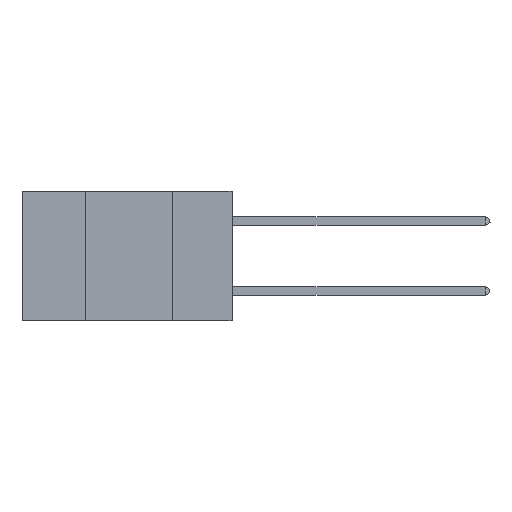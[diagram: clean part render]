
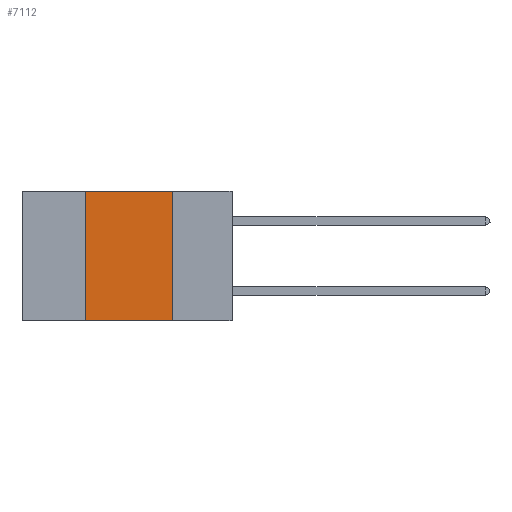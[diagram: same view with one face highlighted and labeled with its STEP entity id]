
A CAD part, left-side view. The second image highlights one B-rep face of the part: STEP entity #7112.
In plain terms, the highlighted planar face has unit normal (-1, 0, 0).
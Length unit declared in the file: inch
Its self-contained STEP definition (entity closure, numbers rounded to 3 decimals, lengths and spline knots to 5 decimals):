
#1137 = ORIENTED_EDGE ( 'NONE', *, *, #18672, .F. ) ;
#1663 = VERTEX_POINT ( 'NONE', #9083 ) ;
#2869 = VERTEX_POINT ( 'NONE', #22920 ) ;
#3941 = DIRECTION ( 'NONE',  ( 1., 0., 0. ) ) ;
#5808 = PLANE ( 'NONE',  #6796 ) ;
#6336 = CARTESIAN_POINT ( 'NONE',  ( 0., 0.42, 0. ) ) ;
#6553 = DIRECTION ( 'NONE',  ( 0., -1., 0. ) ) ;
#6796 = AXIS2_PLACEMENT_3D ( 'NONE', #20015, #3941, #12505 ) ;
#7112 = ADVANCED_FACE ( 'NONE', ( #7330 ), #5808, .F. ) ;
#7273 = LINE ( 'NONE', #19848, #7962 ) ;
#7315 = ORIENTED_EDGE ( 'NONE', *, *, #9141, .F. ) ;
#7330 = FACE_OUTER_BOUND ( 'NONE', #13004, .T. ) ;
#7962 = VECTOR ( 'NONE', #14661, 39.37008 ) ;
#8351 = VERTEX_POINT ( 'NONE', #16168 ) ;
#9083 = CARTESIAN_POINT ( 'NONE',  ( 0., 0.42, -0.37 ) ) ;
#9141 = EDGE_CURVE ( 'NONE', #11763, #8351, #7273, .T. ) ;
#10241 = ORIENTED_EDGE ( 'NONE', *, *, #20338, .T. ) ;
#10461 = EDGE_CURVE ( 'NONE', #1663, #11763, #11507, .T. ) ;
#11011 = CARTESIAN_POINT ( 'NONE',  ( 0., 0.17, 0. ) ) ;
#11507 = LINE ( 'NONE', #15124, #12785 ) ;
#11620 = LINE ( 'NONE', #19012, #22629 ) ;
#11763 = VERTEX_POINT ( 'NONE', #6336 ) ;
#12505 = DIRECTION ( 'NONE',  ( 0., 0., -1. ) ) ;
#12785 = VECTOR ( 'NONE', #18443, 39.37008 ) ;
#13004 = EDGE_LOOP ( 'NONE', ( #1137, #7315, #21924, #10241 ) ) ;
#14289 = DIRECTION ( 'NONE',  ( 0., 0., -1. ) ) ;
#14661 = DIRECTION ( 'NONE',  ( 0., -1., 0. ) ) ;
#15124 = CARTESIAN_POINT ( 'NONE',  ( 0., 0.42, 0. ) ) ;
#16168 = CARTESIAN_POINT ( 'NONE',  ( 0., 0.17, 0. ) ) ;
#16233 = VECTOR ( 'NONE', #14289, 39.37008 ) ;
#18443 = DIRECTION ( 'NONE',  ( 0., 0., 1. ) ) ;
#18672 = EDGE_CURVE ( 'NONE', #8351, #2869, #19938, .T. ) ;
#19012 = CARTESIAN_POINT ( 'NONE',  ( 0., 0.6, -0.37 ) ) ;
#19848 = CARTESIAN_POINT ( 'NONE',  ( 0., 0.6, 0. ) ) ;
#19938 = LINE ( 'NONE', #11011, #16233 ) ;
#20015 = CARTESIAN_POINT ( 'NONE',  ( 0., 0.6, 0. ) ) ;
#20338 = EDGE_CURVE ( 'NONE', #1663, #2869, #11620, .T. ) ;
#21924 = ORIENTED_EDGE ( 'NONE', *, *, #10461, .F. ) ;
#22629 = VECTOR ( 'NONE', #6553, 39.37008 ) ;
#22920 = CARTESIAN_POINT ( 'NONE',  ( 0., 0.17, -0.37 ) ) ;
